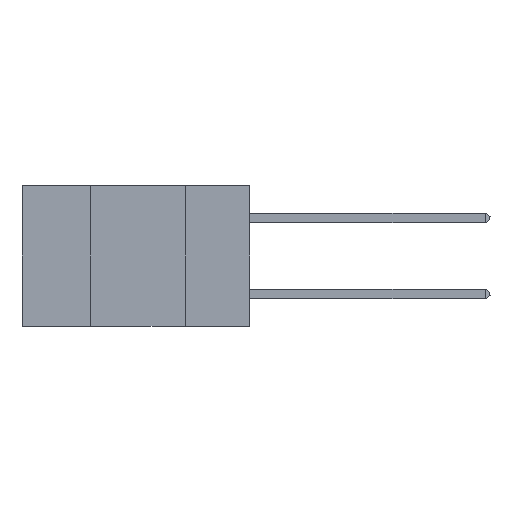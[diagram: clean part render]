
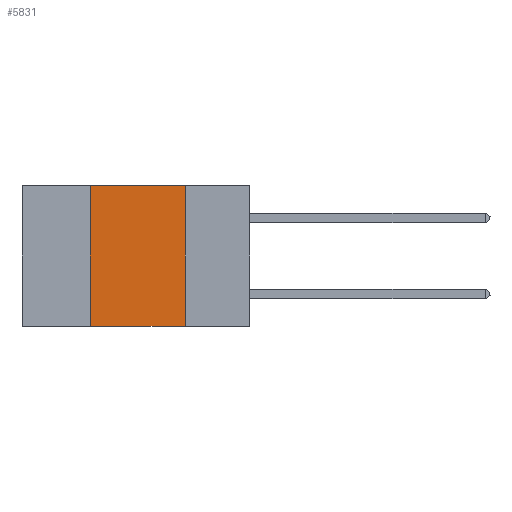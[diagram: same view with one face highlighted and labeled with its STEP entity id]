
A CAD part, left-side view. The second image highlights one B-rep face of the part: STEP entity #5831.
In plain terms, the highlighted planar face has unit normal (-1, 0, 0).
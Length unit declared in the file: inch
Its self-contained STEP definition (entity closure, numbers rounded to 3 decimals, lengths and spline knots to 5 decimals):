
#76 = VERTEX_POINT ( 'NONE', #2160 ) ;
#315 = VECTOR ( 'NONE', #7336, 39.37008 ) ;
#331 = LINE ( 'NONE', #10413, #12059 ) ;
#410 = CARTESIAN_POINT ( 'NONE',  ( 0., 0.17, -0.37 ) ) ;
#1059 = ORIENTED_EDGE ( 'NONE', *, *, #14972, .F. ) ;
#1450 = VECTOR ( 'NONE', #13186, 39.37008 ) ;
#1568 = EDGE_CURVE ( 'NONE', #76, #12329, #331, .T. ) ;
#1888 = EDGE_CURVE ( 'NONE', #11240, #12329, #9071, .T. ) ;
#1992 = CARTESIAN_POINT ( 'NONE',  ( 0., 0.42, -0.37 ) ) ;
#2160 = CARTESIAN_POINT ( 'NONE',  ( 0., 0.17, 0. ) ) ;
#3135 = DIRECTION ( 'NONE',  ( 0., 0., -1. ) ) ;
#3193 = CARTESIAN_POINT ( 'NONE',  ( 0., 0.6, 0. ) ) ;
#4140 = AXIS2_PLACEMENT_3D ( 'NONE', #3193, #5687, #3135 ) ;
#4183 = VERTEX_POINT ( 'NONE', #5600 ) ;
#4480 = PLANE ( 'NONE',  #4140 ) ;
#5600 = CARTESIAN_POINT ( 'NONE',  ( 0., 0.42, 0. ) ) ;
#5687 = DIRECTION ( 'NONE',  ( 1., 0., 0. ) ) ;
#5831 = ADVANCED_FACE ( 'NONE', ( #7776 ), #4480, .F. ) ;
#6716 = DIRECTION ( 'NONE',  ( 0., 0., -1. ) ) ;
#7336 = DIRECTION ( 'NONE',  ( 0., -1., 0. ) ) ;
#7491 = LINE ( 'NONE', #13354, #1450 ) ;
#7776 = FACE_OUTER_BOUND ( 'NONE', #11163, .T. ) ;
#8059 = LINE ( 'NONE', #15387, #14535 ) ;
#9071 = LINE ( 'NONE', #14818, #315 ) ;
#10413 = CARTESIAN_POINT ( 'NONE',  ( 0., 0.17, 0. ) ) ;
#10554 = ORIENTED_EDGE ( 'NONE', *, *, #1568, .F. ) ;
#11163 = EDGE_LOOP ( 'NONE', ( #10554, #14060, #1059, #12217 ) ) ;
#11240 = VERTEX_POINT ( 'NONE', #1992 ) ;
#11413 = DIRECTION ( 'NONE',  ( 0., 0., 1. ) ) ;
#12053 = EDGE_CURVE ( 'NONE', #4183, #76, #7491, .T. ) ;
#12059 = VECTOR ( 'NONE', #6716, 39.37008 ) ;
#12217 = ORIENTED_EDGE ( 'NONE', *, *, #1888, .T. ) ;
#12329 = VERTEX_POINT ( 'NONE', #410 ) ;
#13186 = DIRECTION ( 'NONE',  ( 0., -1., 0. ) ) ;
#13354 = CARTESIAN_POINT ( 'NONE',  ( 0., 0.6, 0. ) ) ;
#14060 = ORIENTED_EDGE ( 'NONE', *, *, #12053, .F. ) ;
#14535 = VECTOR ( 'NONE', #11413, 39.37008 ) ;
#14818 = CARTESIAN_POINT ( 'NONE',  ( 0., 0.6, -0.37 ) ) ;
#14972 = EDGE_CURVE ( 'NONE', #11240, #4183, #8059, .T. ) ;
#15387 = CARTESIAN_POINT ( 'NONE',  ( 0., 0.42, 0. ) ) ;
